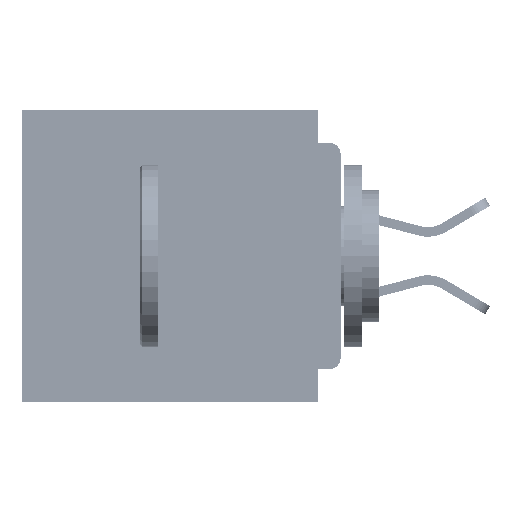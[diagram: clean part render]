
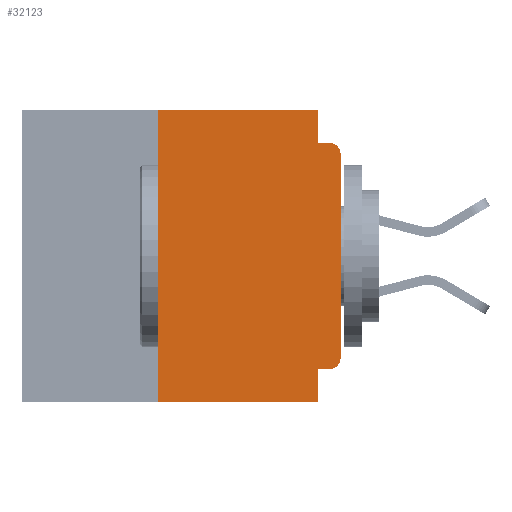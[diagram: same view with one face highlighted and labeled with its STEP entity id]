
A CAD part, left-side view. The second image highlights one B-rep face of the part: STEP entity #32123.
In plain terms, the highlighted planar face has unit normal (-1, 0, 0).
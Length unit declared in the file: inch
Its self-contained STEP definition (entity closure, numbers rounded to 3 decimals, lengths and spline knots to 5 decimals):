
#415 = FACE_OUTER_BOUND ( 'NONE', #66142, .T. ) ;
#853 = DIRECTION ( 'NONE',  ( 0., 0., -1. ) ) ;
#1506 = AXIS2_PLACEMENT_3D ( 'NONE', #66220, #33707, #853 ) ;
#1878 = VERTEX_POINT ( 'NONE', #58269 ) ;
#3119 = VERTEX_POINT ( 'NONE', #14022 ) ;
#3928 = AXIS2_PLACEMENT_3D ( 'NONE', #45043, #12386, #50517 ) ;
#4206 = CARTESIAN_POINT ( 'NONE',  ( 0., 0.031, -0.355 ) ) ;
#4537 = CARTESIAN_POINT ( 'NONE',  ( 0., 0.031, 0. ) ) ;
#4551 = VERTEX_POINT ( 'NONE', #4206 ) ;
#5107 = LINE ( 'NONE', #6455, #61488 ) ;
#6455 = CARTESIAN_POINT ( 'NONE',  ( 0., 0.437, 0. ) ) ;
#6807 = ORIENTED_EDGE ( 'NONE', *, *, #21945, .F. ) ;
#8721 = CARTESIAN_POINT ( 'NONE',  ( 0., 0., 0. ) ) ;
#11024 = EDGE_CURVE ( 'NONE', #47852, #4551, #34350, .T. ) ;
#11917 = CARTESIAN_POINT ( 'NONE',  ( 0., 0.015, -0.045 ) ) ;
#12252 = DIRECTION ( 'NONE',  ( 0., -1., 0. ) ) ;
#12386 = DIRECTION ( 'NONE',  ( 1., 0., 0. ) ) ;
#13355 = EDGE_CURVE ( 'NONE', #47852, #30938, #39162, .T. ) ;
#14022 = CARTESIAN_POINT ( 'NONE',  ( 0., 0.031, -0.4 ) ) ;
#15279 = VECTOR ( 'NONE', #33785, 39.37008 ) ;
#17134 = EDGE_CURVE ( 'NONE', #48408, #3119, #64845, .T. ) ;
#17255 = CARTESIAN_POINT ( 'NONE',  ( 0., 0., -0.045 ) ) ;
#17606 = PLANE ( 'NONE',  #3928 ) ;
#17698 = VECTOR ( 'NONE', #63390, 39.37008 ) ;
#18485 = ORIENTED_EDGE ( 'NONE', *, *, #18864, .F. ) ;
#18864 = EDGE_CURVE ( 'NONE', #48408, #24778, #37326, .T. ) ;
#19179 = DIRECTION ( 'NONE',  ( 0., 0., -1. ) ) ;
#21418 = VECTOR ( 'NONE', #19179, 39.37008 ) ;
#21945 = EDGE_CURVE ( 'NONE', #24778, #55396, #5107, .T. ) ;
#23689 = ORIENTED_EDGE ( 'NONE', *, *, #13355, .T. ) ;
#23823 = DIRECTION ( 'NONE',  ( -1., 0., 0. ) ) ;
#24778 = VERTEX_POINT ( 'NONE', #36721 ) ;
#26025 = VERTEX_POINT ( 'NONE', #27142 ) ;
#27142 = CARTESIAN_POINT ( 'NONE',  ( 0., 0.031, -0.045 ) ) ;
#29139 = VECTOR ( 'NONE', #63404, 39.37008 ) ;
#29449 = ORIENTED_EDGE ( 'NONE', *, *, #17134, .T. ) ;
#30938 = VERTEX_POINT ( 'NONE', #34062 ) ;
#31543 = LINE ( 'NONE', #17255, #15279 ) ;
#32123 = ADVANCED_FACE ( 'NONE', ( #415 ), #17606, .F. ) ;
#33707 = DIRECTION ( 'NONE',  ( -1., 0., 0. ) ) ;
#33785 = DIRECTION ( 'NONE',  ( 0., -1., 0. ) ) ;
#34062 = CARTESIAN_POINT ( 'NONE',  ( 0., 0., -0.34 ) ) ;
#34350 = LINE ( 'NONE', #55357, #47070 ) ;
#34922 = CARTESIAN_POINT ( 'NONE',  ( 0., 0.015, -0.355 ) ) ;
#35372 = DIRECTION ( 'NONE',  ( 0., 0., 1. ) ) ;
#35968 = LINE ( 'NONE', #40917, #21418 ) ;
#36389 = ORIENTED_EDGE ( 'NONE', *, *, #39356, .T. ) ;
#36721 = CARTESIAN_POINT ( 'NONE',  ( 0., 0.25, 0. ) ) ;
#37326 = LINE ( 'NONE', #40806, #62915 ) ;
#39162 = CIRCLE ( 'NONE', #54348, 0.015 ) ;
#39356 = EDGE_CURVE ( 'NONE', #1878, #66405, #67303, .T. ) ;
#39657 = EDGE_CURVE ( 'NONE', #55396, #26025, #61223, .T. ) ;
#40806 = CARTESIAN_POINT ( 'NONE',  ( 0., 0.25, -0.4 ) ) ;
#40917 = CARTESIAN_POINT ( 'NONE',  ( 0., 0.031, -0.4 ) ) ;
#43933 = EDGE_CURVE ( 'NONE', #30938, #1878, #57316, .T. ) ;
#45043 = CARTESIAN_POINT ( 'NONE',  ( 0., 0.437, 0. ) ) ;
#45548 = ORIENTED_EDGE ( 'NONE', *, *, #51426, .F. ) ;
#46954 = CARTESIAN_POINT ( 'NONE',  ( 0., 0.437, -0.4 ) ) ;
#47070 = VECTOR ( 'NONE', #50087, 39.37008 ) ;
#47852 = VERTEX_POINT ( 'NONE', #34922 ) ;
#48408 = VERTEX_POINT ( 'NONE', #63244 ) ;
#49286 = ORIENTED_EDGE ( 'NONE', *, *, #11024, .F. ) ;
#50087 = DIRECTION ( 'NONE',  ( 0., 1., 0. ) ) ;
#50517 = DIRECTION ( 'NONE',  ( 0., 0., -1. ) ) ;
#51426 = EDGE_CURVE ( 'NONE', #26025, #66405, #31543, .T. ) ;
#52396 = DIRECTION ( 'NONE',  ( 0., 0., 1. ) ) ;
#54348 = AXIS2_PLACEMENT_3D ( 'NONE', #56473, #23823, #61928 ) ;
#54803 = ORIENTED_EDGE ( 'NONE', *, *, #43933, .T. ) ;
#55357 = CARTESIAN_POINT ( 'NONE',  ( 0., 0., -0.355 ) ) ;
#55396 = VERTEX_POINT ( 'NONE', #4537 ) ;
#56473 = CARTESIAN_POINT ( 'NONE',  ( 0., 0.015, -0.34 ) ) ;
#57316 = LINE ( 'NONE', #8721, #69964 ) ;
#58269 = CARTESIAN_POINT ( 'NONE',  ( 0., 0., -0.06 ) ) ;
#58918 = ORIENTED_EDGE ( 'NONE', *, *, #39657, .F. ) ;
#61223 = LINE ( 'NONE', #68806, #17698 ) ;
#61488 = VECTOR ( 'NONE', #12252, 39.37008 ) ;
#61928 = DIRECTION ( 'NONE',  ( 0., 0., -1. ) ) ;
#62915 = VECTOR ( 'NONE', #35372, 39.37008 ) ;
#63244 = CARTESIAN_POINT ( 'NONE',  ( 0., 0.25, -0.4 ) ) ;
#63390 = DIRECTION ( 'NONE',  ( 0., 0., -1. ) ) ;
#63404 = DIRECTION ( 'NONE',  ( 0., -1., 0. ) ) ;
#64845 = LINE ( 'NONE', #46954, #29139 ) ;
#66142 = EDGE_LOOP ( 'NONE', ( #54803, #36389, #45548, #58918, #6807, #18485, #29449, #69507, #49286, #23689 ) ) ;
#66220 = CARTESIAN_POINT ( 'NONE',  ( 0., 0.015, -0.06 ) ) ;
#66405 = VERTEX_POINT ( 'NONE', #11917 ) ;
#67303 = CIRCLE ( 'NONE', #1506, 0.015 ) ;
#68806 = CARTESIAN_POINT ( 'NONE',  ( 0., 0.031, 0. ) ) ;
#69507 = ORIENTED_EDGE ( 'NONE', *, *, #69785, .F. ) ;
#69785 = EDGE_CURVE ( 'NONE', #4551, #3119, #35968, .T. ) ;
#69964 = VECTOR ( 'NONE', #52396, 39.37008 ) ;
